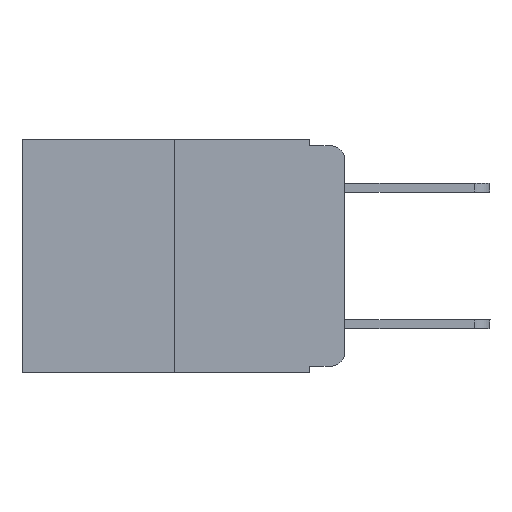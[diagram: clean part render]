
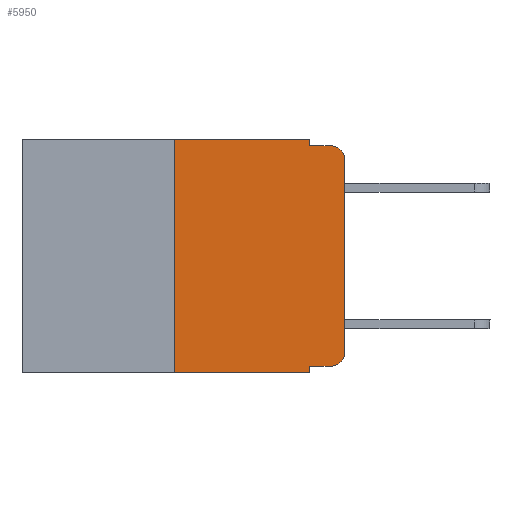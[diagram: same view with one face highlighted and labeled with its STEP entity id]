
A CAD part, left-side view. The second image highlights one B-rep face of the part: STEP entity #5950.
In plain terms, the highlighted planar face has unit normal (-1, 0, 0).
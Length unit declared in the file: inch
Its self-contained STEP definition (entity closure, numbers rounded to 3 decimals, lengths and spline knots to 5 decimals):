
#92 = DIRECTION ( 'NONE',  ( -1., 0., 0. ) ) ;
#225 = ORIENTED_EDGE ( 'NONE', *, *, #7004, .F. ) ;
#386 = CARTESIAN_POINT ( 'NONE',  ( 0., 0.051, 0. ) ) ;
#470 = DIRECTION ( 'NONE',  ( 1., 0., 0. ) ) ;
#676 = CARTESIAN_POINT ( 'NONE',  ( 0., 0., -0.03 ) ) ;
#936 = VECTOR ( 'NONE', #4468, 39.37008 ) ;
#955 = DIRECTION ( 'NONE',  ( 0., 0., 1. ) ) ;
#1251 = AXIS2_PLACEMENT_3D ( 'NONE', #8105, #3162, #8020 ) ;
#1368 = ORIENTED_EDGE ( 'NONE', *, *, #7579, .F. ) ;
#1491 = PLANE ( 'NONE',  #11428 ) ;
#1518 = ORIENTED_EDGE ( 'NONE', *, *, #3133, .T. ) ;
#1749 = ORIENTED_EDGE ( 'NONE', *, *, #8744, .T. ) ;
#1851 = CARTESIAN_POINT ( 'NONE',  ( 0., 0., 0. ) ) ;
#1890 = LINE ( 'NONE', #10717, #9009 ) ;
#1896 = CIRCLE ( 'NONE', #10338, 0.02 ) ;
#2093 = EDGE_LOOP ( 'NONE', ( #3423, #1518, #1368, #6050, #9920, #10518, #7880, #225, #12699, #1749 ) ) ;
#2147 = LINE ( 'NONE', #8233, #2624 ) ;
#2417 = DIRECTION ( 'NONE',  ( 0., 0., -1. ) ) ;
#2624 = VECTOR ( 'NONE', #4247, 39.37008 ) ;
#2804 = EDGE_CURVE ( 'NONE', #3147, #4633, #9686, .T. ) ;
#2872 = CARTESIAN_POINT ( 'NONE',  ( 0., 0.02, -0.03 ) ) ;
#2972 = DIRECTION ( 'NONE',  ( 0., -1., 0. ) ) ;
#3133 = EDGE_CURVE ( 'NONE', #11607, #4391, #1896, .T. ) ;
#3147 = VERTEX_POINT ( 'NONE', #10931 ) ;
#3153 = VECTOR ( 'NONE', #10957, 39.37008 ) ;
#3162 = DIRECTION ( 'NONE',  ( -1., 0., 0. ) ) ;
#3302 = CARTESIAN_POINT ( 'NONE',  ( 0., 0.473, 0. ) ) ;
#3415 = VERTEX_POINT ( 'NONE', #7385 ) ;
#3423 = ORIENTED_EDGE ( 'NONE', *, *, #12328, .T. ) ;
#3522 = LINE ( 'NONE', #7470, #936 ) ;
#4247 = DIRECTION ( 'NONE',  ( 0., -1., 0. ) ) ;
#4348 = VERTEX_POINT ( 'NONE', #7223 ) ;
#4364 = CARTESIAN_POINT ( 'NONE',  ( 0., 0.473, 0. ) ) ;
#4391 = VERTEX_POINT ( 'NONE', #9293 ) ;
#4468 = DIRECTION ( 'NONE',  ( 0., 0., -1. ) ) ;
#4633 = VERTEX_POINT ( 'NONE', #386 ) ;
#4974 = LINE ( 'NONE', #6710, #7013 ) ;
#5555 = LINE ( 'NONE', #7857, #10507 ) ;
#5672 = DIRECTION ( 'NONE',  ( 0., -1., 0. ) ) ;
#5950 = ADVANCED_FACE ( 'NONE', ( #10801 ), #1491, .F. ) ;
#6050 = ORIENTED_EDGE ( 'NONE', *, *, #8895, .F. ) ;
#6058 = EDGE_CURVE ( 'NONE', #7565, #8897, #5555, .T. ) ;
#6117 = VECTOR ( 'NONE', #10216, 39.37008 ) ;
#6289 = LINE ( 'NONE', #7779, #3153 ) ;
#6710 = CARTESIAN_POINT ( 'NONE',  ( 0., 0.051, -0.01 ) ) ;
#7004 = EDGE_CURVE ( 'NONE', #7565, #8859, #1890, .T. ) ;
#7013 = VECTOR ( 'NONE', #5672, 39.37008 ) ;
#7191 = LINE ( 'NONE', #1851, #12156 ) ;
#7223 = CARTESIAN_POINT ( 'NONE',  ( 0., 0.051, -0.01 ) ) ;
#7385 = CARTESIAN_POINT ( 'NONE',  ( 0., 0.25, -0.343 ) ) ;
#7470 = CARTESIAN_POINT ( 'NONE',  ( 0., 0.051, 0. ) ) ;
#7565 = VERTEX_POINT ( 'NONE', #11751 ) ;
#7579 = EDGE_CURVE ( 'NONE', #4348, #4391, #4974, .T. ) ;
#7779 = CARTESIAN_POINT ( 'NONE',  ( 0., 0.25, 0. ) ) ;
#7857 = CARTESIAN_POINT ( 'NONE',  ( 0., 0.051, -0.333 ) ) ;
#7880 = ORIENTED_EDGE ( 'NONE', *, *, #8821, .T. ) ;
#8020 = DIRECTION ( 'NONE',  ( 0., 0., -1. ) ) ;
#8105 = CARTESIAN_POINT ( 'NONE',  ( 0., 0.02, -0.313 ) ) ;
#8233 = CARTESIAN_POINT ( 'NONE',  ( 0., 0.473, -0.343 ) ) ;
#8327 = CARTESIAN_POINT ( 'NONE',  ( 0., 0., -0.313 ) ) ;
#8555 = DIRECTION ( 'NONE',  ( 0., 0., -1. ) ) ;
#8744 = EDGE_CURVE ( 'NONE', #8897, #12703, #11608, .T. ) ;
#8821 = EDGE_CURVE ( 'NONE', #3415, #8859, #2147, .T. ) ;
#8842 = DIRECTION ( 'NONE',  ( 0., 0., -1. ) ) ;
#8859 = VERTEX_POINT ( 'NONE', #11150 ) ;
#8895 = EDGE_CURVE ( 'NONE', #4633, #4348, #3522, .T. ) ;
#8897 = VERTEX_POINT ( 'NONE', #9456 ) ;
#9009 = VECTOR ( 'NONE', #8555, 39.37008 ) ;
#9293 = CARTESIAN_POINT ( 'NONE',  ( 0., 0.02, -0.01 ) ) ;
#9456 = CARTESIAN_POINT ( 'NONE',  ( 0., 0.02, -0.333 ) ) ;
#9686 = LINE ( 'NONE', #3302, #6117 ) ;
#9920 = ORIENTED_EDGE ( 'NONE', *, *, #2804, .F. ) ;
#10216 = DIRECTION ( 'NONE',  ( 0., -1., 0. ) ) ;
#10338 = AXIS2_PLACEMENT_3D ( 'NONE', #2872, #92, #8842 ) ;
#10507 = VECTOR ( 'NONE', #2972, 39.37008 ) ;
#10518 = ORIENTED_EDGE ( 'NONE', *, *, #11728, .F. ) ;
#10717 = CARTESIAN_POINT ( 'NONE',  ( 0., 0.051, 0. ) ) ;
#10801 = FACE_OUTER_BOUND ( 'NONE', #2093, .T. ) ;
#10931 = CARTESIAN_POINT ( 'NONE',  ( 0., 0.25, 0. ) ) ;
#10957 = DIRECTION ( 'NONE',  ( 0., 0., 1. ) ) ;
#11150 = CARTESIAN_POINT ( 'NONE',  ( 0., 0.051, -0.343 ) ) ;
#11428 = AXIS2_PLACEMENT_3D ( 'NONE', #4364, #470, #2417 ) ;
#11607 = VERTEX_POINT ( 'NONE', #676 ) ;
#11608 = CIRCLE ( 'NONE', #1251, 0.02 ) ;
#11728 = EDGE_CURVE ( 'NONE', #3415, #3147, #6289, .T. ) ;
#11751 = CARTESIAN_POINT ( 'NONE',  ( 0., 0.051, -0.333 ) ) ;
#12156 = VECTOR ( 'NONE', #955, 39.37008 ) ;
#12328 = EDGE_CURVE ( 'NONE', #12703, #11607, #7191, .T. ) ;
#12699 = ORIENTED_EDGE ( 'NONE', *, *, #6058, .T. ) ;
#12703 = VERTEX_POINT ( 'NONE', #8327 ) ;
